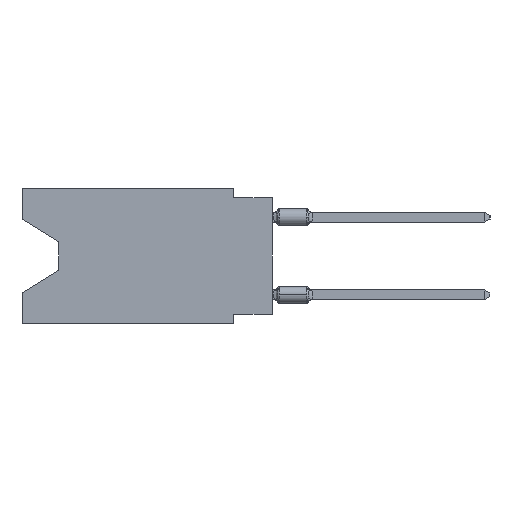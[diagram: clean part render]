
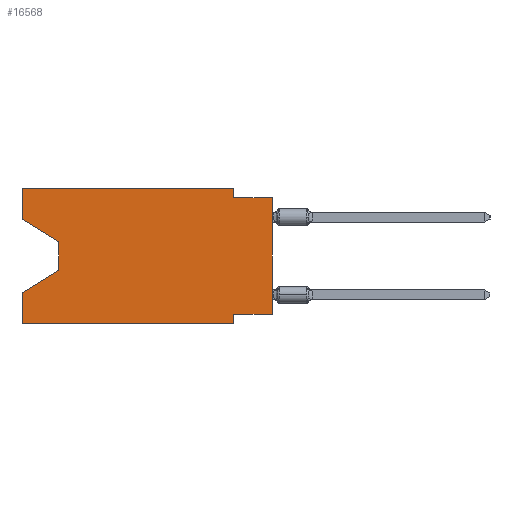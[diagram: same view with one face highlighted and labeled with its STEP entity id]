
A CAD part, left-side view. The second image highlights one B-rep face of the part: STEP entity #16568.
In plain terms, the highlighted planar face has unit normal (-1, 0, 0).
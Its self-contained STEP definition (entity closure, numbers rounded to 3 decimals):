
#2439 = CARTESIAN_POINT ( 'NONE',  ( 0., 13.97, -5.385 ) ) ;
#2520 = CARTESIAN_POINT ( 'NONE',  ( 0., 0., -8.255 ) ) ;
#2726 = VECTOR ( 'NONE', #21913, 1000. ) ;
#3296 = CARTESIAN_POINT ( 'NONE',  ( 0., 16.383, 0. ) ) ;
#3302 = VECTOR ( 'NONE', #32775, 1000. ) ;
#5005 = DIRECTION ( 'NONE',  ( 0., 0., 1. ) ) ;
#5560 = CARTESIAN_POINT ( 'NONE',  ( 0., 16.383, -8.89 ) ) ;
#5626 = VECTOR ( 'NONE', #34438, 1000. ) ;
#5719 = CARTESIAN_POINT ( 'NONE',  ( 0., 13.97, -3.505 ) ) ;
#5959 = VERTEX_POINT ( 'NONE', #13130 ) ;
#6998 = LINE ( 'NONE', #47388, #9849 ) ;
#7590 = LINE ( 'NONE', #10761, #5626 ) ;
#7817 = VERTEX_POINT ( 'NONE', #39002 ) ;
#7931 = VERTEX_POINT ( 'NONE', #2520 ) ;
#8690 = LINE ( 'NONE', #45908, #26544 ) ;
#9280 = ORIENTED_EDGE ( 'NONE', *, *, #42381, .F. ) ;
#9305 = CARTESIAN_POINT ( 'NONE',  ( 0., 16.383, 0. ) ) ;
#9313 = EDGE_CURVE ( 'NONE', #24728, #37918, #26321, .T. ) ;
#9365 = CARTESIAN_POINT ( 'NONE',  ( 0., 0., -8.255 ) ) ;
#9849 = VECTOR ( 'NONE', #24854, 1000. ) ;
#10503 = EDGE_CURVE ( 'NONE', #30708, #5959, #20749, .T. ) ;
#10630 = DIRECTION ( 'NONE',  ( 0., 0., 1. ) ) ;
#10761 = CARTESIAN_POINT ( 'NONE',  ( 0., 16.383, 0. ) ) ;
#11110 = EDGE_CURVE ( 'NONE', #37906, #46157, #36333, .T. ) ;
#11908 = EDGE_CURVE ( 'NONE', #37918, #7817, #48255, .T. ) ;
#12339 = LINE ( 'NONE', #23590, #19792 ) ;
#12359 = DIRECTION ( 'NONE',  ( 0., 0., 1. ) ) ;
#12612 = CARTESIAN_POINT ( 'NONE',  ( 0., 2.54, 0. ) ) ;
#12770 = ORIENTED_EDGE ( 'NONE', *, *, #26972, .T. ) ;
#13115 = EDGE_CURVE ( 'NONE', #7931, #16390, #43137, .T. ) ;
#13123 = CARTESIAN_POINT ( 'NONE',  ( 0., 2.54, -0.635 ) ) ;
#13130 = CARTESIAN_POINT ( 'NONE',  ( 0., 2.54, -8.89 ) ) ;
#13975 = CARTESIAN_POINT ( 'NONE',  ( 0., 0., -0.635 ) ) ;
#14763 = AXIS2_PLACEMENT_3D ( 'NONE', #28679, #47535, #44351 ) ;
#14859 = LINE ( 'NONE', #18534, #44797 ) ;
#15573 = DIRECTION ( 'NONE',  ( 0., -0.855, -0.519 ) ) ;
#16390 = VERTEX_POINT ( 'NONE', #16688 ) ;
#16568 = ADVANCED_FACE ( 'NONE', ( #17905 ), #43860, .F. ) ;
#16688 = CARTESIAN_POINT ( 'NONE',  ( 0., 2.54, -8.255 ) ) ;
#17058 = DIRECTION ( 'NONE',  ( 0., -1., 0. ) ) ;
#17416 = LINE ( 'NONE', #43625, #36207 ) ;
#17905 = FACE_OUTER_BOUND ( 'NONE', #42391, .T. ) ;
#18534 = CARTESIAN_POINT ( 'NONE',  ( 0., 16.383, -2.038 ) ) ;
#18979 = CARTESIAN_POINT ( 'NONE',  ( 0., 2.54, 0. ) ) ;
#19792 = VECTOR ( 'NONE', #5005, 1000. ) ;
#20159 = ORIENTED_EDGE ( 'NONE', *, *, #40443, .T. ) ;
#20749 = LINE ( 'NONE', #43269, #43510 ) ;
#21913 = DIRECTION ( 'NONE',  ( 0., 0., -1. ) ) ;
#23590 = CARTESIAN_POINT ( 'NONE',  ( 0., 16.383, 0. ) ) ;
#23903 = CARTESIAN_POINT ( 'NONE',  ( 0., 16.383, -2.038 ) ) ;
#24461 = LINE ( 'NONE', #2439, #3302 ) ;
#24728 = VERTEX_POINT ( 'NONE', #12612 ) ;
#24854 = DIRECTION ( 'NONE',  ( 0., 0., -1. ) ) ;
#26321 = LINE ( 'NONE', #18979, #2726 ) ;
#26544 = VECTOR ( 'NONE', #12359, 1000. ) ;
#26558 = ORIENTED_EDGE ( 'NONE', *, *, #13115, .F. ) ;
#26778 = ORIENTED_EDGE ( 'NONE', *, *, #34542, .T. ) ;
#26972 = EDGE_CURVE ( 'NONE', #38835, #41823, #24461, .T. ) ;
#28679 = CARTESIAN_POINT ( 'NONE',  ( 0., 16.383, 0. ) ) ;
#29623 = DIRECTION ( 'NONE',  ( 0., -1., 0. ) ) ;
#29820 = ORIENTED_EDGE ( 'NONE', *, *, #11908, .F. ) ;
#30708 = VERTEX_POINT ( 'NONE', #5560 ) ;
#31278 = EDGE_CURVE ( 'NONE', #39145, #38835, #6998, .T. ) ;
#31832 = VECTOR ( 'NONE', #29623, 1000. ) ;
#31959 = ORIENTED_EDGE ( 'NONE', *, *, #11110, .F. ) ;
#32775 = DIRECTION ( 'NONE',  ( 0., 0.855, -0.519 ) ) ;
#33205 = ORIENTED_EDGE ( 'NONE', *, *, #10503, .T. ) ;
#34438 = DIRECTION ( 'NONE',  ( 0., -1., 0. ) ) ;
#34542 = EDGE_CURVE ( 'NONE', #7931, #7817, #8690, .T. ) ;
#35536 = DIRECTION ( 'NONE',  ( 0., 1., 0. ) ) ;
#36207 = VECTOR ( 'NONE', #47065, 1000. ) ;
#36333 = LINE ( 'NONE', #3296, #44316 ) ;
#37386 = ORIENTED_EDGE ( 'NONE', *, *, #31278, .T. ) ;
#37906 = VERTEX_POINT ( 'NONE', #23903 ) ;
#37918 = VERTEX_POINT ( 'NONE', #13123 ) ;
#38835 = VERTEX_POINT ( 'NONE', #40751 ) ;
#39002 = CARTESIAN_POINT ( 'NONE',  ( 0., 0., -0.635 ) ) ;
#39145 = VERTEX_POINT ( 'NONE', #5719 ) ;
#39643 = EDGE_CURVE ( 'NONE', #46157, #24728, #7590, .T. ) ;
#40443 = EDGE_CURVE ( 'NONE', #37906, #39145, #14859, .T. ) ;
#40713 = EDGE_CURVE ( 'NONE', #16390, #5959, #17416, .T. ) ;
#40751 = CARTESIAN_POINT ( 'NONE',  ( 0., 13.97, -5.385 ) ) ;
#41690 = ORIENTED_EDGE ( 'NONE', *, *, #40713, .F. ) ;
#41823 = VERTEX_POINT ( 'NONE', #45224 ) ;
#42381 = EDGE_CURVE ( 'NONE', #30708, #41823, #12339, .T. ) ;
#42391 = EDGE_LOOP ( 'NONE', ( #20159, #37386, #12770, #9280, #33205, #41690, #26558, #26778, #29820, #43871, #42702, #31959 ) ) ;
#42702 = ORIENTED_EDGE ( 'NONE', *, *, #39643, .F. ) ;
#43137 = LINE ( 'NONE', #9365, #45819 ) ;
#43269 = CARTESIAN_POINT ( 'NONE',  ( 0., 16.383, -8.89 ) ) ;
#43510 = VECTOR ( 'NONE', #17058, 1000. ) ;
#43625 = CARTESIAN_POINT ( 'NONE',  ( 0., 2.54, -8.89 ) ) ;
#43860 = PLANE ( 'NONE',  #14763 ) ;
#43871 = ORIENTED_EDGE ( 'NONE', *, *, #9313, .F. ) ;
#44316 = VECTOR ( 'NONE', #10630, 1000. ) ;
#44351 = DIRECTION ( 'NONE',  ( 0., 0., -1. ) ) ;
#44797 = VECTOR ( 'NONE', #15573, 1000. ) ;
#45224 = CARTESIAN_POINT ( 'NONE',  ( 0., 16.383, -6.852 ) ) ;
#45819 = VECTOR ( 'NONE', #35536, 1000. ) ;
#45908 = CARTESIAN_POINT ( 'NONE',  ( 0., 0., 0. ) ) ;
#46157 = VERTEX_POINT ( 'NONE', #9305 ) ;
#47065 = DIRECTION ( 'NONE',  ( 0., 0., -1. ) ) ;
#47388 = CARTESIAN_POINT ( 'NONE',  ( 0., 13.97, -3.505 ) ) ;
#47535 = DIRECTION ( 'NONE',  ( 1., 0., 0. ) ) ;
#48255 = LINE ( 'NONE', #13975, #31832 ) ;
